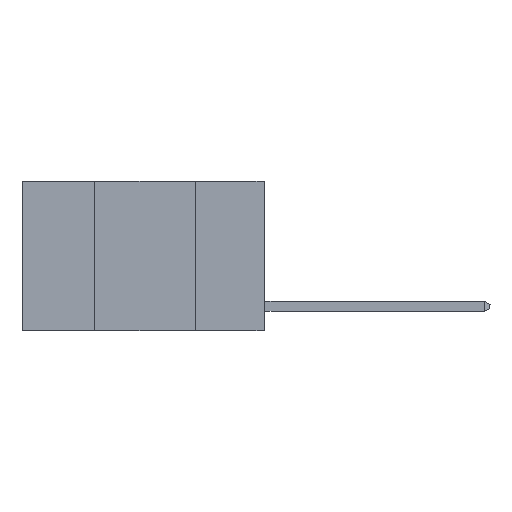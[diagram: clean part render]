
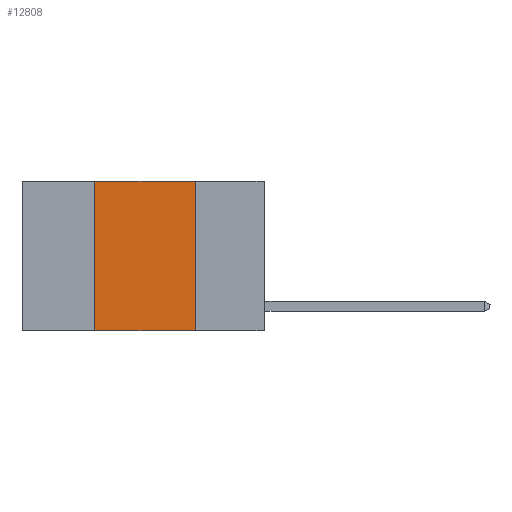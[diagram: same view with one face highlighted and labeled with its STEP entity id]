
A CAD part, left-side view. The second image highlights one B-rep face of the part: STEP entity #12808.
In plain terms, the highlighted planar face has unit normal (-1, 0, 0).
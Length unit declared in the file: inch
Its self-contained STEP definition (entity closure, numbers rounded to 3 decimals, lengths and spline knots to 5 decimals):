
#711 = CARTESIAN_POINT ( 'NONE',  ( 0., 0.17, 0. ) ) ;
#1229 = ORIENTED_EDGE ( 'NONE', *, *, #4082, .F. ) ;
#2963 = ORIENTED_EDGE ( 'NONE', *, *, #13123, .F. ) ;
#3312 = VERTEX_POINT ( 'NONE', #9285 ) ;
#4082 = EDGE_CURVE ( 'NONE', #13259, #3312, #9412, .T. ) ;
#4187 = EDGE_LOOP ( 'NONE', ( #1229, #2963, #7701, #21441 ) ) ;
#4814 = LINE ( 'NONE', #17084, #13947 ) ;
#4866 = CARTESIAN_POINT ( 'NONE',  ( 0., 0.42, 0. ) ) ;
#7086 = DIRECTION ( 'NONE',  ( 0., 0., 1. ) ) ;
#7169 = CARTESIAN_POINT ( 'NONE',  ( 0., 0.6, 0. ) ) ;
#7701 = ORIENTED_EDGE ( 'NONE', *, *, #12805, .F. ) ;
#7731 = DIRECTION ( 'NONE',  ( 0., -1., 0. ) ) ;
#8869 = PLANE ( 'NONE',  #19927 ) ;
#9285 = CARTESIAN_POINT ( 'NONE',  ( 0., 0.17, -0.37 ) ) ;
#9412 = LINE ( 'NONE', #711, #17450 ) ;
#11179 = VECTOR ( 'NONE', #7731, 39.37008 ) ;
#12805 = EDGE_CURVE ( 'NONE', #16436, #13871, #13414, .T. ) ;
#12808 = ADVANCED_FACE ( 'NONE', ( #14542 ), #8869, .F. ) ;
#13123 = EDGE_CURVE ( 'NONE', #13871, #13259, #4814, .T. ) ;
#13194 = DIRECTION ( 'NONE',  ( 0., 0., -1. ) ) ;
#13259 = VERTEX_POINT ( 'NONE', #14033 ) ;
#13414 = LINE ( 'NONE', #15939, #16788 ) ;
#13871 = VERTEX_POINT ( 'NONE', #4866 ) ;
#13947 = VECTOR ( 'NONE', #15218, 39.37008 ) ;
#14033 = CARTESIAN_POINT ( 'NONE',  ( 0., 0.17, 0. ) ) ;
#14525 = DIRECTION ( 'NONE',  ( 0., 0., -1. ) ) ;
#14542 = FACE_OUTER_BOUND ( 'NONE', #4187, .T. ) ;
#15053 = LINE ( 'NONE', #21907, #11179 ) ;
#15218 = DIRECTION ( 'NONE',  ( 0., -1., 0. ) ) ;
#15939 = CARTESIAN_POINT ( 'NONE',  ( 0., 0.42, 0. ) ) ;
#16071 = EDGE_CURVE ( 'NONE', #16436, #3312, #15053, .T. ) ;
#16436 = VERTEX_POINT ( 'NONE', #18915 ) ;
#16567 = DIRECTION ( 'NONE',  ( 1., 0., 0. ) ) ;
#16788 = VECTOR ( 'NONE', #7086, 39.37008 ) ;
#17084 = CARTESIAN_POINT ( 'NONE',  ( 0., 0.6, 0. ) ) ;
#17450 = VECTOR ( 'NONE', #13194, 39.37008 ) ;
#18915 = CARTESIAN_POINT ( 'NONE',  ( 0., 0.42, -0.37 ) ) ;
#19927 = AXIS2_PLACEMENT_3D ( 'NONE', #7169, #16567, #14525 ) ;
#21441 = ORIENTED_EDGE ( 'NONE', *, *, #16071, .T. ) ;
#21907 = CARTESIAN_POINT ( 'NONE',  ( 0., 0.6, -0.37 ) ) ;
